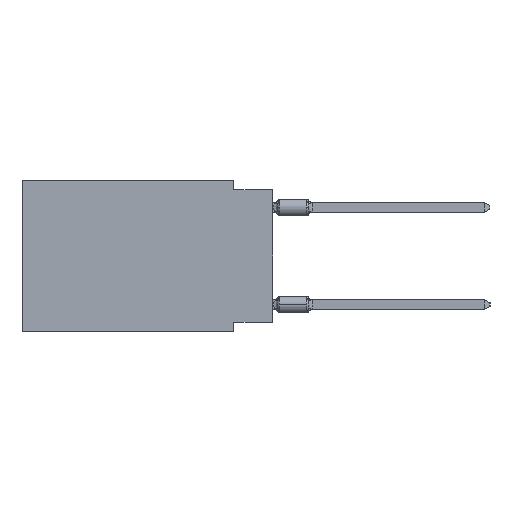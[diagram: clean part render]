
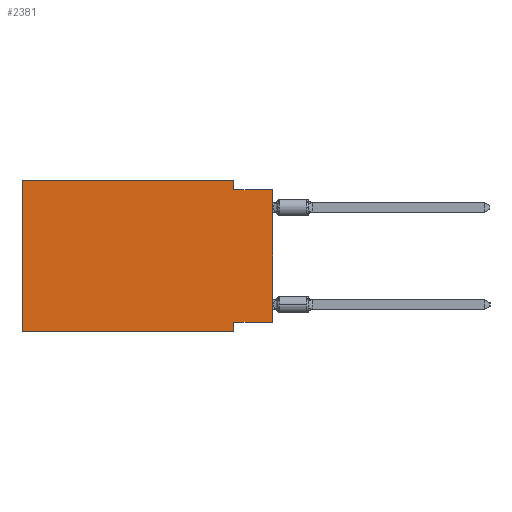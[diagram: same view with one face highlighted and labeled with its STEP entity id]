
A CAD part, left-side view. The second image highlights one B-rep face of the part: STEP entity #2381.
In plain terms, the highlighted planar face has unit normal (-1, 0, 0).
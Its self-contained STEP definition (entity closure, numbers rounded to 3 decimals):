
#265 = CARTESIAN_POINT ( 'NONE',  ( 0., 0., -9.271 ) ) ;
#429 = DIRECTION ( 'NONE',  ( 0., 1., 0. ) ) ;
#1049 = DIRECTION ( 'NONE',  ( 0., 0., -1. ) ) ;
#1501 = DIRECTION ( 'NONE',  ( 0., 0., -1. ) ) ;
#2381 = ADVANCED_FACE ( 'NONE', ( #27546 ), #10372, .F. ) ;
#2487 = DIRECTION ( 'NONE',  ( 1., 0., 0. ) ) ;
#2637 = DIRECTION ( 'NONE',  ( 0., 0., -1. ) ) ;
#2873 = CARTESIAN_POINT ( 'NONE',  ( 0., 2.54, -9.271 ) ) ;
#3245 = VECTOR ( 'NONE', #28495, 1000. ) ;
#3463 = EDGE_CURVE ( 'NONE', #14513, #28472, #24731, .T. ) ;
#3498 = ORIENTED_EDGE ( 'NONE', *, *, #23669, .F. ) ;
#4296 = CARTESIAN_POINT ( 'NONE',  ( 0., 2.54, -9.906 ) ) ;
#5788 = VERTEX_POINT ( 'NONE', #22143 ) ;
#6993 = VERTEX_POINT ( 'NONE', #26320 ) ;
#7362 = EDGE_CURVE ( 'NONE', #5788, #22075, #25641, .T. ) ;
#7630 = VECTOR ( 'NONE', #1049, 1000. ) ;
#8211 = CARTESIAN_POINT ( 'NONE',  ( 0., 16.383, -9.906 ) ) ;
#8804 = CARTESIAN_POINT ( 'NONE',  ( 0., 16.383, -9.906 ) ) ;
#10372 = PLANE ( 'NONE',  #13048 ) ;
#10441 = VECTOR ( 'NONE', #25311, 1000. ) ;
#12060 = ORIENTED_EDGE ( 'NONE', *, *, #7362, .T. ) ;
#12404 = VECTOR ( 'NONE', #17426, 1000. ) ;
#12602 = LINE ( 'NONE', #265, #25592 ) ;
#13048 = AXIS2_PLACEMENT_3D ( 'NONE', #17629, #2487, #2637 ) ;
#13233 = CARTESIAN_POINT ( 'NONE',  ( 0., 0., -0.635 ) ) ;
#13546 = CARTESIAN_POINT ( 'NONE',  ( 0., 2.54, 0. ) ) ;
#13566 = EDGE_LOOP ( 'NONE', ( #12060, #25111, #17067, #23533, #29575, #20031, #32220, #3498 ) ) ;
#13957 = VERTEX_POINT ( 'NONE', #27338 ) ;
#14513 = VERTEX_POINT ( 'NONE', #2873 ) ;
#14950 = LINE ( 'NONE', #29980, #12404 ) ;
#15250 = CARTESIAN_POINT ( 'NONE',  ( 0., 0., 0. ) ) ;
#15724 = LINE ( 'NONE', #13233, #29855 ) ;
#17067 = ORIENTED_EDGE ( 'NONE', *, *, #29069, .F. ) ;
#17426 = DIRECTION ( 'NONE',  ( 0., 0., 1. ) ) ;
#17516 = VERTEX_POINT ( 'NONE', #8804 ) ;
#17629 = CARTESIAN_POINT ( 'NONE',  ( 0., 16.383, 0. ) ) ;
#17937 = LINE ( 'NONE', #8211, #3245 ) ;
#18780 = VECTOR ( 'NONE', #22732, 1000. ) ;
#18981 = LINE ( 'NONE', #13546, #7630 ) ;
#20031 = ORIENTED_EDGE ( 'NONE', *, *, #24476, .T. ) ;
#20058 = CARTESIAN_POINT ( 'NONE',  ( 0., 2.54, -9.906 ) ) ;
#21909 = EDGE_CURVE ( 'NONE', #6993, #22075, #15724, .T. ) ;
#22075 = VERTEX_POINT ( 'NONE', #26113 ) ;
#22143 = CARTESIAN_POINT ( 'NONE',  ( 0., 0., -9.271 ) ) ;
#22732 = DIRECTION ( 'NONE',  ( 0., -1., 0. ) ) ;
#23533 = ORIENTED_EDGE ( 'NONE', *, *, #31035, .F. ) ;
#23669 = EDGE_CURVE ( 'NONE', #5788, #14513, #12602, .T. ) ;
#24476 = EDGE_CURVE ( 'NONE', #17516, #28472, #17937, .T. ) ;
#24731 = LINE ( 'NONE', #4296, #27377 ) ;
#25111 = ORIENTED_EDGE ( 'NONE', *, *, #21909, .F. ) ;
#25311 = DIRECTION ( 'NONE',  ( 0., 0., 1. ) ) ;
#25376 = LINE ( 'NONE', #30828, #18780 ) ;
#25592 = VECTOR ( 'NONE', #429, 1000. ) ;
#25641 = LINE ( 'NONE', #15250, #10441 ) ;
#26113 = CARTESIAN_POINT ( 'NONE',  ( 0., 0., -0.635 ) ) ;
#26320 = CARTESIAN_POINT ( 'NONE',  ( 0., 2.54, -0.635 ) ) ;
#27338 = CARTESIAN_POINT ( 'NONE',  ( 0., 2.54, 0. ) ) ;
#27377 = VECTOR ( 'NONE', #1501, 1000. ) ;
#27546 = FACE_OUTER_BOUND ( 'NONE', #13566, .T. ) ;
#27954 = DIRECTION ( 'NONE',  ( 0., -1., 0. ) ) ;
#27987 = CARTESIAN_POINT ( 'NONE',  ( 0., 16.383, 0. ) ) ;
#28472 = VERTEX_POINT ( 'NONE', #20058 ) ;
#28495 = DIRECTION ( 'NONE',  ( 0., -1., 0. ) ) ;
#29069 = EDGE_CURVE ( 'NONE', #13957, #6993, #18981, .T. ) ;
#29575 = ORIENTED_EDGE ( 'NONE', *, *, #29680, .F. ) ;
#29680 = EDGE_CURVE ( 'NONE', #17516, #29698, #14950, .T. ) ;
#29698 = VERTEX_POINT ( 'NONE', #27987 ) ;
#29855 = VECTOR ( 'NONE', #27954, 1000. ) ;
#29980 = CARTESIAN_POINT ( 'NONE',  ( 0., 16.383, 0. ) ) ;
#30828 = CARTESIAN_POINT ( 'NONE',  ( 0., 16.383, 0. ) ) ;
#31035 = EDGE_CURVE ( 'NONE', #29698, #13957, #25376, .T. ) ;
#32220 = ORIENTED_EDGE ( 'NONE', *, *, #3463, .F. ) ;
